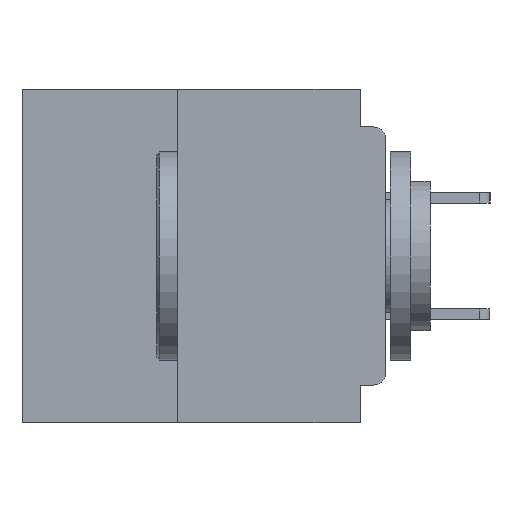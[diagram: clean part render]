
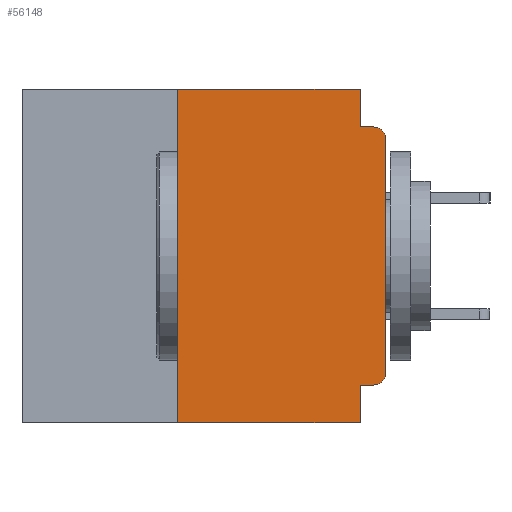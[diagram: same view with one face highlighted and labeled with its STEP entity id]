
A CAD part, left-side view. The second image highlights one B-rep face of the part: STEP entity #56148.
In plain terms, the highlighted planar face has unit normal (-1, 0, 0).
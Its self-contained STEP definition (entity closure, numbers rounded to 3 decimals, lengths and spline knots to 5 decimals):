
#448 = DIRECTION ( 'NONE',  ( 0., 0., -1. ) ) ;
#2210 = CIRCLE ( 'NONE', #26002, 0.015 ) ;
#4211 = VERTEX_POINT ( 'NONE', #4983 ) ;
#4570 = VERTEX_POINT ( 'NONE', #53213 ) ;
#4947 = CARTESIAN_POINT ( 'NONE',  ( 0., 0.25, -0.4 ) ) ;
#4983 = CARTESIAN_POINT ( 'NONE',  ( 0., 0.25, 0. ) ) ;
#5223 = CARTESIAN_POINT ( 'NONE',  ( 0., 0.25, -0.4 ) ) ;
#7409 = VECTOR ( 'NONE', #23796, 39.37008 ) ;
#7980 = CARTESIAN_POINT ( 'NONE',  ( 0., 0.015, -0.045 ) ) ;
#9544 = VERTEX_POINT ( 'NONE', #46590 ) ;
#9740 = LINE ( 'NONE', #10629, #48682 ) ;
#10629 = CARTESIAN_POINT ( 'NONE',  ( 0., 0., -0.045 ) ) ;
#10784 = VERTEX_POINT ( 'NONE', #31378 ) ;
#11107 = CARTESIAN_POINT ( 'NONE',  ( 0., 0., 0. ) ) ;
#12011 = CARTESIAN_POINT ( 'NONE',  ( 0., 0.031, -0.355 ) ) ;
#12974 = CARTESIAN_POINT ( 'NONE',  ( 0., 0.031, -0.4 ) ) ;
#13204 = VERTEX_POINT ( 'NONE', #15360 ) ;
#13491 = CARTESIAN_POINT ( 'NONE',  ( 0., 0.031, 0. ) ) ;
#13701 = LINE ( 'NONE', #26692, #42581 ) ;
#14030 = ORIENTED_EDGE ( 'NONE', *, *, #21355, .F. ) ;
#14380 = LINE ( 'NONE', #4947, #26395 ) ;
#14661 = VECTOR ( 'NONE', #46658, 39.37008 ) ;
#15360 = CARTESIAN_POINT ( 'NONE',  ( 0., 0., -0.06 ) ) ;
#15672 = VERTEX_POINT ( 'NONE', #49923 ) ;
#15758 = DIRECTION ( 'NONE',  ( 0., -1., 0. ) ) ;
#16498 = CARTESIAN_POINT ( 'NONE',  ( 0., 0.015, -0.34 ) ) ;
#16880 = VECTOR ( 'NONE', #50109, 39.37008 ) ;
#19619 = ORIENTED_EDGE ( 'NONE', *, *, #47085, .F. ) ;
#21346 = EDGE_CURVE ( 'NONE', #13204, #42332, #2210, .T. ) ;
#21355 = EDGE_CURVE ( 'NONE', #60912, #4211, #14380, .T. ) ;
#21659 = DIRECTION ( 'NONE',  ( 0., 0., -1. ) ) ;
#23519 = AXIS2_PLACEMENT_3D ( 'NONE', #16498, #52005, #21659 ) ;
#23796 = DIRECTION ( 'NONE',  ( 0., 0., -1. ) ) ;
#24550 = VERTEX_POINT ( 'NONE', #12011 ) ;
#25613 = DIRECTION ( 'NONE',  ( 0., 0., 1. ) ) ;
#26002 = AXIS2_PLACEMENT_3D ( 'NONE', #30756, #49159, #35870 ) ;
#26395 = VECTOR ( 'NONE', #25613, 39.37008 ) ;
#26692 = CARTESIAN_POINT ( 'NONE',  ( 0., 0.437, -0.4 ) ) ;
#26867 = ORIENTED_EDGE ( 'NONE', *, *, #32073, .F. ) ;
#28268 = LINE ( 'NONE', #11107, #14661 ) ;
#28467 = ORIENTED_EDGE ( 'NONE', *, *, #40054, .T. ) ;
#29322 = CARTESIAN_POINT ( 'NONE',  ( 0., 0.015, -0.355 ) ) ;
#30197 = LINE ( 'NONE', #12974, #60182 ) ;
#30493 = LINE ( 'NONE', #65059, #16880 ) ;
#30756 = CARTESIAN_POINT ( 'NONE',  ( 0., 0.015, -0.06 ) ) ;
#31283 = DIRECTION ( 'NONE',  ( 1., 0., 0. ) ) ;
#31378 = CARTESIAN_POINT ( 'NONE',  ( 0., 0., -0.34 ) ) ;
#32073 = EDGE_CURVE ( 'NONE', #56629, #24550, #51543, .T. ) ;
#32780 = CARTESIAN_POINT ( 'NONE',  ( 0., 0., -0.355 ) ) ;
#34049 = ORIENTED_EDGE ( 'NONE', *, *, #47833, .T. ) ;
#34366 = EDGE_CURVE ( 'NONE', #24550, #4570, #30197, .T. ) ;
#35870 = DIRECTION ( 'NONE',  ( 0., 0., -1. ) ) ;
#38142 = VECTOR ( 'NONE', #42880, 39.37008 ) ;
#38242 = EDGE_CURVE ( 'NONE', #15672, #42332, #9740, .T. ) ;
#39529 = ORIENTED_EDGE ( 'NONE', *, *, #53152, .F. ) ;
#40054 = EDGE_CURVE ( 'NONE', #56629, #10784, #50739, .T. ) ;
#40285 = ORIENTED_EDGE ( 'NONE', *, *, #21346, .T. ) ;
#41186 = CARTESIAN_POINT ( 'NONE',  ( 0., 0.437, 0. ) ) ;
#42332 = VERTEX_POINT ( 'NONE', #7980 ) ;
#42581 = VECTOR ( 'NONE', #62002, 39.37008 ) ;
#42698 = EDGE_CURVE ( 'NONE', #10784, #13204, #28268, .T. ) ;
#42880 = DIRECTION ( 'NONE',  ( 0., 1., 0. ) ) ;
#43431 = DIRECTION ( 'NONE',  ( 0., 0., -1. ) ) ;
#43738 = EDGE_LOOP ( 'NONE', ( #52107, #40285, #58440, #19619, #39529, #14030, #34049, #60840, #26867, #28467 ) ) ;
#46590 = CARTESIAN_POINT ( 'NONE',  ( 0., 0.031, 0. ) ) ;
#46658 = DIRECTION ( 'NONE',  ( 0., 0., 1. ) ) ;
#47085 = EDGE_CURVE ( 'NONE', #9544, #15672, #61417, .T. ) ;
#47833 = EDGE_CURVE ( 'NONE', #60912, #4570, #13701, .T. ) ;
#48682 = VECTOR ( 'NONE', #15758, 39.37008 ) ;
#49159 = DIRECTION ( 'NONE',  ( -1., 0., 0. ) ) ;
#49923 = CARTESIAN_POINT ( 'NONE',  ( 0., 0.031, -0.045 ) ) ;
#50109 = DIRECTION ( 'NONE',  ( 0., -1., 0. ) ) ;
#50739 = CIRCLE ( 'NONE', #23519, 0.015 ) ;
#51334 = PLANE ( 'NONE',  #65854 ) ;
#51543 = LINE ( 'NONE', #32780, #38142 ) ;
#52005 = DIRECTION ( 'NONE',  ( -1., 0., 0. ) ) ;
#52107 = ORIENTED_EDGE ( 'NONE', *, *, #42698, .T. ) ;
#53152 = EDGE_CURVE ( 'NONE', #4211, #9544, #30493, .T. ) ;
#53213 = CARTESIAN_POINT ( 'NONE',  ( 0., 0.031, -0.4 ) ) ;
#56148 = ADVANCED_FACE ( 'NONE', ( #64047 ), #51334, .F. ) ;
#56629 = VERTEX_POINT ( 'NONE', #29322 ) ;
#58440 = ORIENTED_EDGE ( 'NONE', *, *, #38242, .F. ) ;
#60182 = VECTOR ( 'NONE', #43431, 39.37008 ) ;
#60840 = ORIENTED_EDGE ( 'NONE', *, *, #34366, .F. ) ;
#60912 = VERTEX_POINT ( 'NONE', #5223 ) ;
#61417 = LINE ( 'NONE', #13491, #7409 ) ;
#62002 = DIRECTION ( 'NONE',  ( 0., -1., 0. ) ) ;
#64047 = FACE_OUTER_BOUND ( 'NONE', #43738, .T. ) ;
#65059 = CARTESIAN_POINT ( 'NONE',  ( 0., 0.437, 0. ) ) ;
#65854 = AXIS2_PLACEMENT_3D ( 'NONE', #41186, #31283, #448 ) ;
